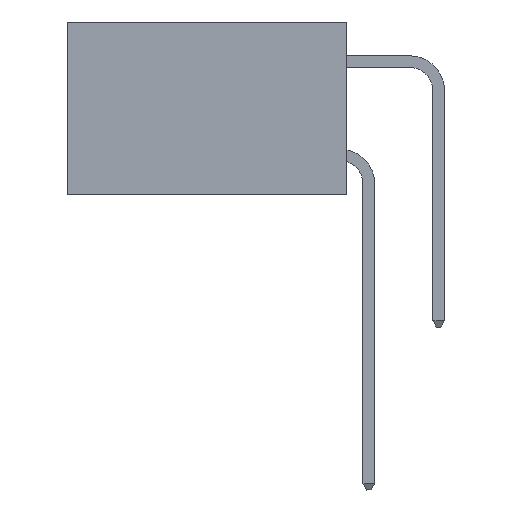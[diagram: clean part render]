
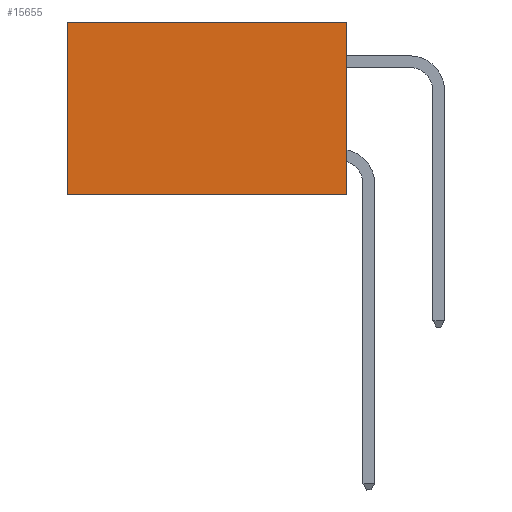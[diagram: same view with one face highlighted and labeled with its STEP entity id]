
A CAD part, left-side view. The second image highlights one B-rep face of the part: STEP entity #15655.
In plain terms, the highlighted planar face has unit normal (-1, 0, 0).
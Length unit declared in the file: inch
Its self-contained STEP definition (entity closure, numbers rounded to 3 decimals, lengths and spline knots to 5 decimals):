
#474 = DIRECTION ( 'NONE',  ( 1., 0., 0. ) ) ;
#787 = VECTOR ( 'NONE', #12652, 39.37008 ) ;
#3316 = FACE_OUTER_BOUND ( 'NONE', #30524, .T. ) ;
#3795 = CARTESIAN_POINT ( 'NONE',  ( 0.2875, 0., 0. ) ) ;
#3997 = ORIENTED_EDGE ( 'NONE', *, *, #16271, .F. ) ;
#4138 = CARTESIAN_POINT ( 'NONE',  ( 0.2875, 0., 0. ) ) ;
#4216 = LINE ( 'NONE', #14095, #15741 ) ;
#4328 = CARTESIAN_POINT ( 'NONE',  ( 0.2875, 0.6, -0.37 ) ) ;
#5935 = ORIENTED_EDGE ( 'NONE', *, *, #17708, .T. ) ;
#5955 = LINE ( 'NONE', #4138, #787 ) ;
#6784 = DIRECTION ( 'NONE',  ( 0., 1., 0. ) ) ;
#8900 = DIRECTION ( 'NONE',  ( 0., 0., -1. ) ) ;
#9051 = EDGE_CURVE ( 'NONE', #28601, #26734, #25849, .T. ) ;
#9827 = VECTOR ( 'NONE', #6784, 39.37008 ) ;
#11679 = LINE ( 'NONE', #16990, #9827 ) ;
#12305 = PLANE ( 'NONE',  #26332 ) ;
#12652 = DIRECTION ( 'NONE',  ( 0., 1., 0. ) ) ;
#13443 = CARTESIAN_POINT ( 'NONE',  ( 0.2875, 0., -0.37 ) ) ;
#14076 = EDGE_CURVE ( 'NONE', #24487, #26734, #11679, .T. ) ;
#14095 = CARTESIAN_POINT ( 'NONE',  ( 0.2875, 0., 0. ) ) ;
#15655 = ADVANCED_FACE ( 'NONE', ( #3316 ), #12305, .F. ) ;
#15741 = VECTOR ( 'NONE', #8900, 39.37008 ) ;
#16271 = EDGE_CURVE ( 'NONE', #20577, #24487, #4216, .T. ) ;
#16990 = CARTESIAN_POINT ( 'NONE',  ( 0.2875, 0., -0.37 ) ) ;
#17708 = EDGE_CURVE ( 'NONE', #20577, #28601, #5955, .T. ) ;
#17759 = ORIENTED_EDGE ( 'NONE', *, *, #9051, .T. ) ;
#18858 = DIRECTION ( 'NONE',  ( 0., 0., -1. ) ) ;
#20577 = VERTEX_POINT ( 'NONE', #3795 ) ;
#21589 = DIRECTION ( 'NONE',  ( 0., 0., -1. ) ) ;
#23585 = ORIENTED_EDGE ( 'NONE', *, *, #14076, .F. ) ;
#24487 = VERTEX_POINT ( 'NONE', #13443 ) ;
#25849 = LINE ( 'NONE', #27170, #29072 ) ;
#26332 = AXIS2_PLACEMENT_3D ( 'NONE', #27365, #474, #21589 ) ;
#26734 = VERTEX_POINT ( 'NONE', #4328 ) ;
#27170 = CARTESIAN_POINT ( 'NONE',  ( 0.2875, 0.6, 0. ) ) ;
#27365 = CARTESIAN_POINT ( 'NONE',  ( 0.2875, 0., 0. ) ) ;
#28601 = VERTEX_POINT ( 'NONE', #35574 ) ;
#29072 = VECTOR ( 'NONE', #18858, 39.37008 ) ;
#30524 = EDGE_LOOP ( 'NONE', ( #17759, #23585, #3997, #5935 ) ) ;
#35574 = CARTESIAN_POINT ( 'NONE',  ( 0.2875, 0.6, 0. ) ) ;
